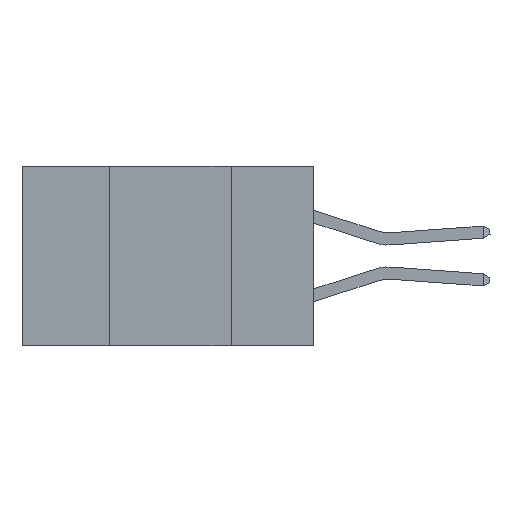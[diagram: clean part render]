
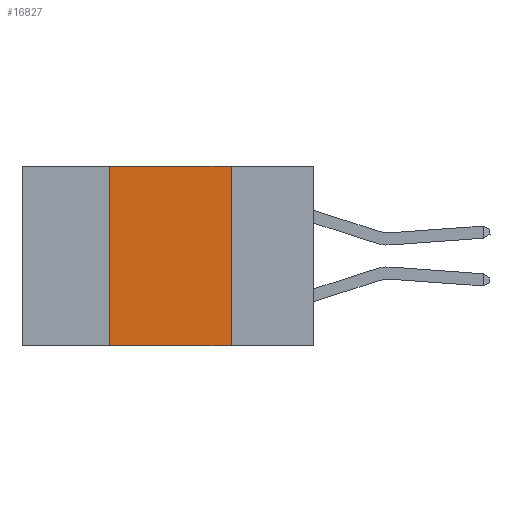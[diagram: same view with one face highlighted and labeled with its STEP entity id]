
A CAD part, left-side view. The second image highlights one B-rep face of the part: STEP entity #16827.
In plain terms, the highlighted planar face has unit normal (-1, 0, 0).
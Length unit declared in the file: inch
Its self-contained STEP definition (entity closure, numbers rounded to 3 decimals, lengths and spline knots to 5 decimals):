
#1989 = FACE_OUTER_BOUND ( 'NONE', #23496, .T. ) ;
#3302 = EDGE_CURVE ( 'NONE', #17518, #37988, #5229, .T. ) ;
#4382 = LINE ( 'NONE', #10472, #24804 ) ;
#5040 = DIRECTION ( 'NONE',  ( 0., 0., -1. ) ) ;
#5229 = LINE ( 'NONE', #20413, #12074 ) ;
#5248 = DIRECTION ( 'NONE',  ( 1., 0., 0. ) ) ;
#9394 = VERTEX_POINT ( 'NONE', #39470 ) ;
#9960 = LINE ( 'NONE', #19289, #22906 ) ;
#10149 = CARTESIAN_POINT ( 'NONE',  ( 0., 0.6, -0.37 ) ) ;
#10472 = CARTESIAN_POINT ( 'NONE',  ( 0., 0.42, 0. ) ) ;
#10557 = DIRECTION ( 'NONE',  ( 0., -1., 0. ) ) ;
#10989 = EDGE_CURVE ( 'NONE', #9394, #17518, #9960, .T. ) ;
#11136 = VECTOR ( 'NONE', #10557, 39.37008 ) ;
#12074 = VECTOR ( 'NONE', #32831, 39.37008 ) ;
#13505 = DIRECTION ( 'NONE',  ( 0., 0., 1. ) ) ;
#15472 = ORIENTED_EDGE ( 'NONE', *, *, #29083, .T. ) ;
#16701 = CARTESIAN_POINT ( 'NONE',  ( 0., 0.17, 0. ) ) ;
#16827 = ADVANCED_FACE ( 'NONE', ( #1989 ), #17793, .F. ) ;
#17437 = ORIENTED_EDGE ( 'NONE', *, *, #26705, .F. ) ;
#17518 = VERTEX_POINT ( 'NONE', #16701 ) ;
#17793 = PLANE ( 'NONE',  #37078 ) ;
#19289 = CARTESIAN_POINT ( 'NONE',  ( 0., 0.6, 0. ) ) ;
#19485 = LINE ( 'NONE', #10149, #11136 ) ;
#20413 = CARTESIAN_POINT ( 'NONE',  ( 0., 0.17, 0. ) ) ;
#20984 = VERTEX_POINT ( 'NONE', #37777 ) ;
#22906 = VECTOR ( 'NONE', #40041, 39.37008 ) ;
#23496 = EDGE_LOOP ( 'NONE', ( #35490, #37980, #17437, #15472 ) ) ;
#24804 = VECTOR ( 'NONE', #13505, 39.37008 ) ;
#26705 = EDGE_CURVE ( 'NONE', #20984, #9394, #4382, .T. ) ;
#26937 = CARTESIAN_POINT ( 'NONE',  ( 0., 0.6, 0. ) ) ;
#29083 = EDGE_CURVE ( 'NONE', #20984, #37988, #19485, .T. ) ;
#32831 = DIRECTION ( 'NONE',  ( 0., 0., -1. ) ) ;
#35490 = ORIENTED_EDGE ( 'NONE', *, *, #3302, .F. ) ;
#37061 = CARTESIAN_POINT ( 'NONE',  ( 0., 0.17, -0.37 ) ) ;
#37078 = AXIS2_PLACEMENT_3D ( 'NONE', #26937, #5248, #5040 ) ;
#37777 = CARTESIAN_POINT ( 'NONE',  ( 0., 0.42, -0.37 ) ) ;
#37980 = ORIENTED_EDGE ( 'NONE', *, *, #10989, .F. ) ;
#37988 = VERTEX_POINT ( 'NONE', #37061 ) ;
#39470 = CARTESIAN_POINT ( 'NONE',  ( 0., 0.42, 0. ) ) ;
#40041 = DIRECTION ( 'NONE',  ( 0., -1., 0. ) ) ;
